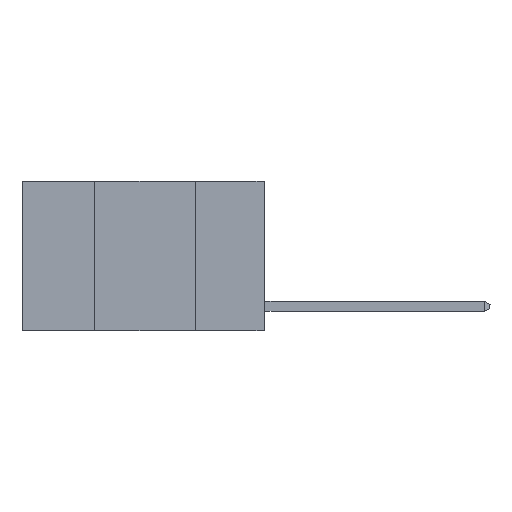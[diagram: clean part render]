
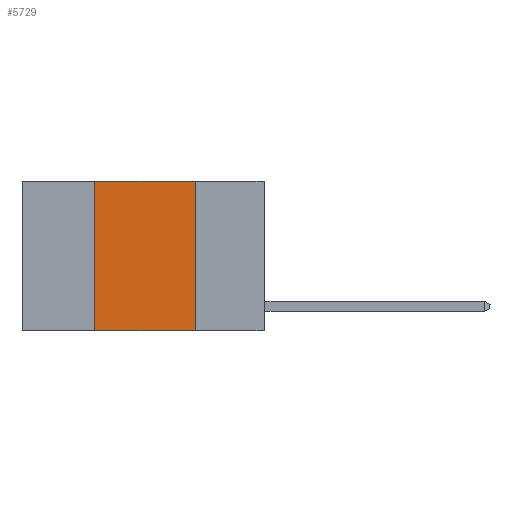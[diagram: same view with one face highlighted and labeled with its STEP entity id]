
A CAD part, left-side view. The second image highlights one B-rep face of the part: STEP entity #5729.
In plain terms, the highlighted planar face has unit normal (-1, 0, 0).
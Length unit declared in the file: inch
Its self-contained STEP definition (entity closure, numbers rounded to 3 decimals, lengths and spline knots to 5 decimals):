
#1172 = VECTOR ( 'NONE', #14161, 39.37008 ) ;
#1182 = CARTESIAN_POINT ( 'NONE',  ( 0., 0.17, -0.37 ) ) ;
#1594 = DIRECTION ( 'NONE',  ( 0., 0., 1. ) ) ;
#1668 = CARTESIAN_POINT ( 'NONE',  ( 0., 0.6, -0.37 ) ) ;
#2276 = CARTESIAN_POINT ( 'NONE',  ( 0., 0.17, 0. ) ) ;
#2375 = CARTESIAN_POINT ( 'NONE',  ( 0., 0.6, 0. ) ) ;
#2485 = FACE_OUTER_BOUND ( 'NONE', #12504, .T. ) ;
#2492 = DIRECTION ( 'NONE',  ( 0., -1., 0. ) ) ;
#2955 = DIRECTION ( 'NONE',  ( 0., -1., 0. ) ) ;
#3107 = EDGE_CURVE ( 'NONE', #12567, #16444, #16532, .T. ) ;
#3730 = LINE ( 'NONE', #1668, #15794 ) ;
#3815 = CARTESIAN_POINT ( 'NONE',  ( 0., 0.42, 0. ) ) ;
#4850 = ORIENTED_EDGE ( 'NONE', *, *, #6594, .T. ) ;
#4903 = CARTESIAN_POINT ( 'NONE',  ( 0., 0.42, -0.37 ) ) ;
#4963 = VECTOR ( 'NONE', #2492, 39.37008 ) ;
#5174 = VERTEX_POINT ( 'NONE', #1182 ) ;
#5548 = ORIENTED_EDGE ( 'NONE', *, *, #3107, .F. ) ;
#5550 = CARTESIAN_POINT ( 'NONE',  ( 0., 0.17, 0. ) ) ;
#5729 = ADVANCED_FACE ( 'NONE', ( #2485 ), #16779, .F. ) ;
#6594 = EDGE_CURVE ( 'NONE', #12567, #5174, #3730, .T. ) ;
#7467 = ORIENTED_EDGE ( 'NONE', *, *, #8094, .F. ) ;
#7608 = VERTEX_POINT ( 'NONE', #5550 ) ;
#7696 = LINE ( 'NONE', #2375, #4963 ) ;
#7826 = EDGE_CURVE ( 'NONE', #7608, #5174, #15963, .T. ) ;
#8094 = EDGE_CURVE ( 'NONE', #16444, #7608, #7696, .T. ) ;
#9921 = DIRECTION ( 'NONE',  ( 1., 0., 0. ) ) ;
#11044 = VECTOR ( 'NONE', #1594, 39.37008 ) ;
#11098 = AXIS2_PLACEMENT_3D ( 'NONE', #13930, #9921, #13994 ) ;
#12504 = EDGE_LOOP ( 'NONE', ( #14078, #7467, #5548, #4850 ) ) ;
#12567 = VERTEX_POINT ( 'NONE', #4903 ) ;
#13930 = CARTESIAN_POINT ( 'NONE',  ( 0., 0.6, 0. ) ) ;
#13994 = DIRECTION ( 'NONE',  ( 0., 0., -1. ) ) ;
#14078 = ORIENTED_EDGE ( 'NONE', *, *, #7826, .F. ) ;
#14161 = DIRECTION ( 'NONE',  ( 0., 0., -1. ) ) ;
#15054 = CARTESIAN_POINT ( 'NONE',  ( 0., 0.42, 0. ) ) ;
#15794 = VECTOR ( 'NONE', #2955, 39.37008 ) ;
#15963 = LINE ( 'NONE', #2276, #1172 ) ;
#16444 = VERTEX_POINT ( 'NONE', #3815 ) ;
#16532 = LINE ( 'NONE', #15054, #11044 ) ;
#16779 = PLANE ( 'NONE',  #11098 ) ;
